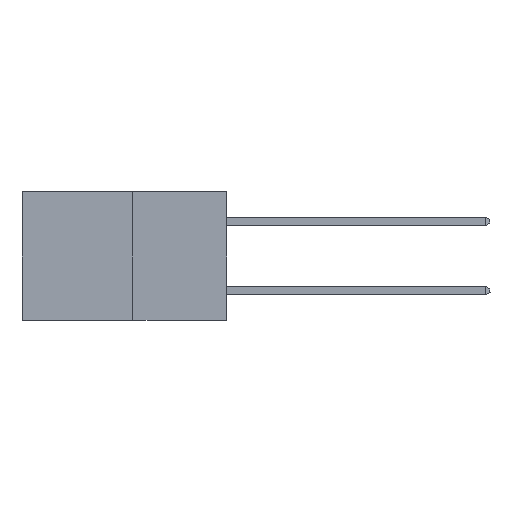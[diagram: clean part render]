
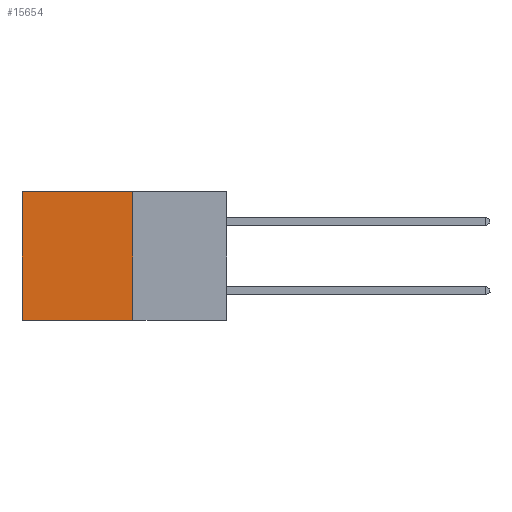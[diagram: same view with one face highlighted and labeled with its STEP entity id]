
A CAD part, left-side view. The second image highlights one B-rep face of the part: STEP entity #15654.
In plain terms, the highlighted planar face has unit normal (-1, 0, 0).
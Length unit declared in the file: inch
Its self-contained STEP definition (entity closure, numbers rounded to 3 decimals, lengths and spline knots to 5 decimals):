
#1986 = AXIS2_PLACEMENT_3D ( 'NONE', #15344, #5159, #17033 ) ;
#3397 = PLANE ( 'NONE',  #1986 ) ;
#4110 = DIRECTION ( 'NONE',  ( 0., 0., -1. ) ) ;
#4542 = FACE_OUTER_BOUND ( 'NONE', #18434, .T. ) ;
#4606 = VECTOR ( 'NONE', #12735, 39.37008 ) ;
#4615 = ORIENTED_EDGE ( 'NONE', *, *, #10356, .F. ) ;
#5159 = DIRECTION ( 'NONE',  ( 1., 0., 0. ) ) ;
#5702 = EDGE_CURVE ( 'NONE', #15718, #10035, #18974, .T. ) ;
#5986 = ORIENTED_EDGE ( 'NONE', *, *, #12422, .T. ) ;
#6089 = CARTESIAN_POINT ( 'NONE',  ( 0.277, 0.59, -0.37 ) ) ;
#6092 = LINE ( 'NONE', #17697, #10652 ) ;
#6794 = ORIENTED_EDGE ( 'NONE', *, *, #5702, .F. ) ;
#7562 = ORIENTED_EDGE ( 'NONE', *, *, #19678, .T. ) ;
#9225 = LINE ( 'NONE', #11042, #4606 ) ;
#9738 = VERTEX_POINT ( 'NONE', #10505 ) ;
#9787 = CARTESIAN_POINT ( 'NONE',  ( 0.277, 0.59, 0. ) ) ;
#10035 = VERTEX_POINT ( 'NONE', #6089 ) ;
#10356 = EDGE_CURVE ( 'NONE', #9738, #15718, #6092, .T. ) ;
#10505 = CARTESIAN_POINT ( 'NONE',  ( 0.277, 0.27, 0. ) ) ;
#10652 = VECTOR ( 'NONE', #4110, 39.37008 ) ;
#11042 = CARTESIAN_POINT ( 'NONE',  ( 0.277, 0.59, -0.37 ) ) ;
#11205 = DIRECTION ( 'NONE',  ( 0., 1., 0. ) ) ;
#12196 = VECTOR ( 'NONE', #11205, 39.37008 ) ;
#12208 = CARTESIAN_POINT ( 'NONE',  ( 0.277, 0.27, -0.37 ) ) ;
#12422 = EDGE_CURVE ( 'NONE', #9738, #21734, #16114, .T. ) ;
#12735 = DIRECTION ( 'NONE',  ( 0., 0., -1. ) ) ;
#15344 = CARTESIAN_POINT ( 'NONE',  ( 0.277, 0.27, -0.37 ) ) ;
#15654 = ADVANCED_FACE ( 'NONE', ( #4542 ), #3397, .F. ) ;
#15718 = VERTEX_POINT ( 'NONE', #12208 ) ;
#16114 = LINE ( 'NONE', #16198, #12196 ) ;
#16198 = CARTESIAN_POINT ( 'NONE',  ( 0.277, 0.27, 0. ) ) ;
#17033 = DIRECTION ( 'NONE',  ( 0., 0., -1. ) ) ;
#17697 = CARTESIAN_POINT ( 'NONE',  ( 0.277, 0.27, -0.37 ) ) ;
#18034 = DIRECTION ( 'NONE',  ( 0., 1., 0. ) ) ;
#18144 = CARTESIAN_POINT ( 'NONE',  ( 0.277, 0.27, -0.37 ) ) ;
#18434 = EDGE_LOOP ( 'NONE', ( #7562, #6794, #4615, #5986 ) ) ;
#18448 = VECTOR ( 'NONE', #18034, 39.37008 ) ;
#18974 = LINE ( 'NONE', #18144, #18448 ) ;
#19678 = EDGE_CURVE ( 'NONE', #21734, #10035, #9225, .T. ) ;
#21734 = VERTEX_POINT ( 'NONE', #9787 ) ;
